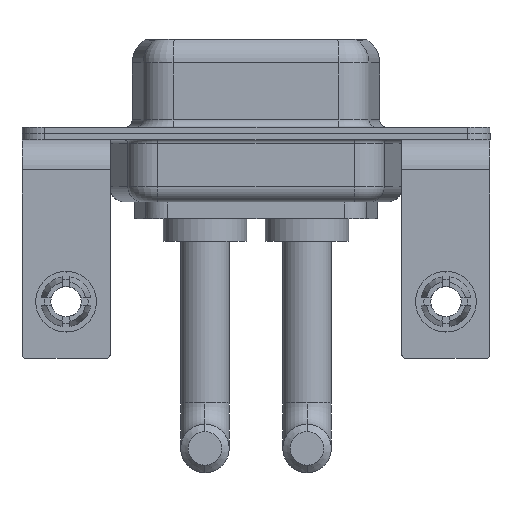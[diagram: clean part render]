
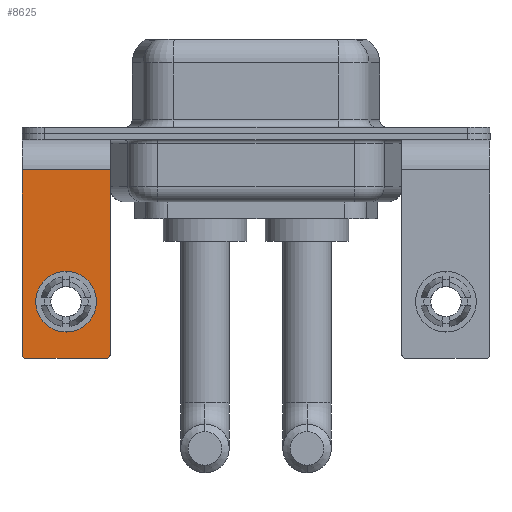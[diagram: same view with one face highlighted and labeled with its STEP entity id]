
A CAD part, front view. The second image highlights one B-rep face of the part: STEP entity #8625.
In plain terms, the highlighted planar face has unit normal (0, -1, 0).
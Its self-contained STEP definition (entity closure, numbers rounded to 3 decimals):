
#705 = CARTESIAN_POINT ( 'NONE',  ( 0., -6.25, -11.07 ) ) ;
#821 = EDGE_CURVE ( 'NONE', #4690, #11841, #13982, .T. ) ;
#868 = EDGE_CURVE ( 'NONE', #11797, #12957, #9261, .T. ) ;
#949 = VERTEX_POINT ( 'NONE', #2728 ) ;
#1092 = CARTESIAN_POINT ( 'NONE',  ( 2.9, -6.25, -2.4 ) ) ;
#1095 = CARTESIAN_POINT ( 'NONE',  ( 0., -6.25, -9.07 ) ) ;
#1109 = EDGE_CURVE ( 'NONE', #5904, #11841, #5731, .T. ) ;
#1261 = ORIENTED_EDGE ( 'NONE', *, *, #8152, .T. ) ;
#1403 = AXIS2_PLACEMENT_3D ( 'NONE', #9054, #5812, #7057 ) ;
#1756 = ORIENTED_EDGE ( 'NONE', *, *, #11087, .T. ) ;
#1938 = FACE_OUTER_BOUND ( 'NONE', #14453, .T. ) ;
#2099 = CARTESIAN_POINT ( 'NONE',  ( -2.65, -6.25, -14.8 ) ) ;
#2124 = CARTESIAN_POINT ( 'NONE',  ( 2.65, -6.25, -14.8 ) ) ;
#2673 = DIRECTION ( 'NONE',  ( -1., 0., 0. ) ) ;
#2728 = CARTESIAN_POINT ( 'NONE',  ( 0., -6.25, -13.07 ) ) ;
#2814 = VECTOR ( 'NONE', #11974, 1000. ) ;
#2877 = DIRECTION ( 'NONE',  ( 0., 0., -1. ) ) ;
#2985 = CARTESIAN_POINT ( 'NONE',  ( -2.9, -6.25, -2.4 ) ) ;
#3081 = ORIENTED_EDGE ( 'NONE', *, *, #4008, .F. ) ;
#3430 = VECTOR ( 'NONE', #2673, 1000. ) ;
#3658 = DIRECTION ( 'NONE',  ( 0., 0., 1. ) ) ;
#4008 = EDGE_CURVE ( 'NONE', #5904, #12957, #9599, .T. ) ;
#4310 = PLANE ( 'NONE',  #5880 ) ;
#4395 = ORIENTED_EDGE ( 'NONE', *, *, #13856, .T. ) ;
#4417 = LINE ( 'NONE', #1092, #10188 ) ;
#4690 = VERTEX_POINT ( 'NONE', #5160 ) ;
#4911 = CARTESIAN_POINT ( 'NONE',  ( 2.65, -6.25, -14.55 ) ) ;
#5051 = DIRECTION ( 'NONE',  ( 0., 0., 1. ) ) ;
#5160 = CARTESIAN_POINT ( 'NONE',  ( 2.9, -6.25, -2.4 ) ) ;
#5336 = CARTESIAN_POINT ( 'NONE',  ( 2.9, -6.25, -2.4 ) ) ;
#5595 = DIRECTION ( 'NONE',  ( -1., 0., 0. ) ) ;
#5731 = CIRCLE ( 'NONE', #13245, 0.25 ) ;
#5812 = DIRECTION ( 'NONE',  ( 0., 1., 0. ) ) ;
#5874 = DIRECTION ( 'NONE',  ( 0., -1., 0. ) ) ;
#5880 = AXIS2_PLACEMENT_3D ( 'NONE', #5336, #12246, #6594 ) ;
#5904 = VERTEX_POINT ( 'NONE', #2124 ) ;
#5984 = CARTESIAN_POINT ( 'NONE',  ( -2.65, -6.25, -14.55 ) ) ;
#6135 = CIRCLE ( 'NONE', #1403, 2. ) ;
#6183 = CARTESIAN_POINT ( 'NONE',  ( -2.9, -6.25, -2.4 ) ) ;
#6216 = CARTESIAN_POINT ( 'NONE',  ( 2.9, -6.25, -14.8 ) ) ;
#6310 = LINE ( 'NONE', #2985, #2814 ) ;
#6594 = DIRECTION ( 'NONE',  ( 0., 0., 1. ) ) ;
#6999 = ORIENTED_EDGE ( 'NONE', *, *, #868, .T. ) ;
#7057 = DIRECTION ( 'NONE',  ( 0., 0., 1. ) ) ;
#7549 = ORIENTED_EDGE ( 'NONE', *, *, #821, .F. ) ;
#7754 = FACE_BOUND ( 'NONE', #7876, .T. ) ;
#7876 = EDGE_LOOP ( 'NONE', ( #1756, #11405 ) ) ;
#8071 = EDGE_CURVE ( 'NONE', #10988, #949, #11755, .T. ) ;
#8152 = EDGE_CURVE ( 'NONE', #12022, #11797, #6310, .T. ) ;
#8625 = ADVANCED_FACE ( 'NONE', ( #7754, #1938 ), #4310, .F. ) ;
#8669 = DIRECTION ( 'NONE',  ( 0., 1., 0. ) ) ;
#9054 = CARTESIAN_POINT ( 'NONE',  ( 0., -6.25, -11.07 ) ) ;
#9261 = CIRCLE ( 'NONE', #13940, 0.25 ) ;
#9410 = AXIS2_PLACEMENT_3D ( 'NONE', #705, #8669, #5051 ) ;
#9511 = CARTESIAN_POINT ( 'NONE',  ( 2.9, -6.25, -2.4 ) ) ;
#9599 = LINE ( 'NONE', #6216, #3430 ) ;
#10188 = VECTOR ( 'NONE', #5595, 1000. ) ;
#10988 = VERTEX_POINT ( 'NONE', #1095 ) ;
#11087 = EDGE_CURVE ( 'NONE', #949, #10988, #6135, .T. ) ;
#11139 = CARTESIAN_POINT ( 'NONE',  ( 2.9, -6.25, -14.55 ) ) ;
#11405 = ORIENTED_EDGE ( 'NONE', *, *, #8071, .T. ) ;
#11721 = CARTESIAN_POINT ( 'NONE',  ( -2.9, -6.25, -14.55 ) ) ;
#11755 = CIRCLE ( 'NONE', #9410, 2. ) ;
#11797 = VERTEX_POINT ( 'NONE', #11721 ) ;
#11841 = VERTEX_POINT ( 'NONE', #11139 ) ;
#11974 = DIRECTION ( 'NONE',  ( 0., 0., -1. ) ) ;
#12022 = VERTEX_POINT ( 'NONE', #6183 ) ;
#12056 = ORIENTED_EDGE ( 'NONE', *, *, #1109, .T. ) ;
#12246 = DIRECTION ( 'NONE',  ( 0., 1., 0. ) ) ;
#12525 = VECTOR ( 'NONE', #2877, 1000. ) ;
#12737 = DIRECTION ( 'NONE',  ( 0., -1., 0. ) ) ;
#12810 = DIRECTION ( 'NONE',  ( 0., 0., 1. ) ) ;
#12957 = VERTEX_POINT ( 'NONE', #2099 ) ;
#13245 = AXIS2_PLACEMENT_3D ( 'NONE', #4911, #5874, #3658 ) ;
#13856 = EDGE_CURVE ( 'NONE', #4690, #12022, #4417, .T. ) ;
#13940 = AXIS2_PLACEMENT_3D ( 'NONE', #5984, #12737, #12810 ) ;
#13982 = LINE ( 'NONE', #9511, #12525 ) ;
#14453 = EDGE_LOOP ( 'NONE', ( #1261, #6999, #3081, #12056, #7549, #4395 ) ) ;
